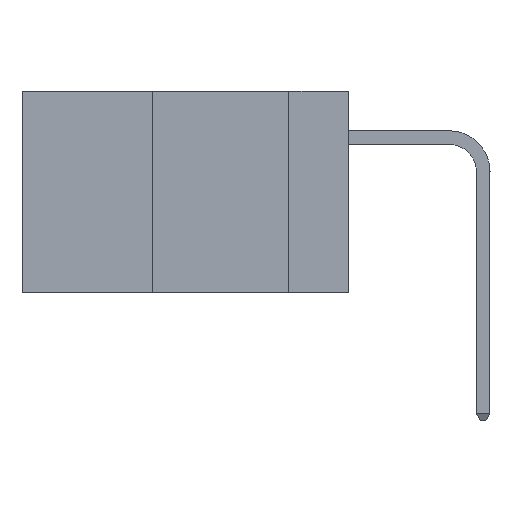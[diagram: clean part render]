
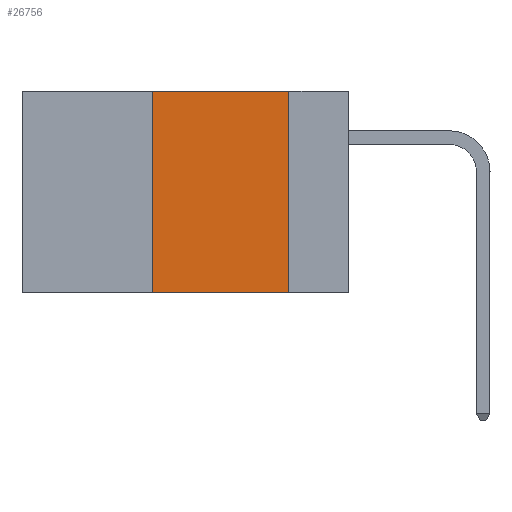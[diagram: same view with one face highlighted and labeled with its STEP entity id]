
A CAD part, left-side view. The second image highlights one B-rep face of the part: STEP entity #26756.
In plain terms, the highlighted planar face has unit normal (-1, 0, 0).
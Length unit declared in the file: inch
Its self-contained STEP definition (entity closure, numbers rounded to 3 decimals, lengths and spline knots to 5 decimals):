
#107 = CARTESIAN_POINT ( 'NONE',  ( 0., 0.11, 0. ) ) ;
#817 = VECTOR ( 'NONE', #8602, 39.37008 ) ;
#1219 = LINE ( 'NONE', #19257, #31223 ) ;
#3360 = VERTEX_POINT ( 'NONE', #4359 ) ;
#4359 = CARTESIAN_POINT ( 'NONE',  ( 0., 0.11, -0.37 ) ) ;
#5262 = CARTESIAN_POINT ( 'NONE',  ( 0., 0.6, -0.37 ) ) ;
#5291 = CARTESIAN_POINT ( 'NONE',  ( 0., 0.6, 0. ) ) ;
#7704 = EDGE_CURVE ( 'NONE', #17013, #25837, #30000, .T. ) ;
#8229 = DIRECTION ( 'NONE',  ( 0., 0., -1. ) ) ;
#8472 = ORIENTED_EDGE ( 'NONE', *, *, #32264, .T. ) ;
#8602 = DIRECTION ( 'NONE',  ( 0., -1., 0. ) ) ;
#11655 = VECTOR ( 'NONE', #19543, 39.37008 ) ;
#12601 = ORIENTED_EDGE ( 'NONE', *, *, #7704, .F. ) ;
#12730 = VERTEX_POINT ( 'NONE', #15192 ) ;
#12817 = CARTESIAN_POINT ( 'NONE',  ( 0., 0.11, 0. ) ) ;
#12995 = VECTOR ( 'NONE', #20111, 39.37008 ) ;
#13951 = EDGE_LOOP ( 'NONE', ( #27179, #12601, #33499, #8472 ) ) ;
#15192 = CARTESIAN_POINT ( 'NONE',  ( 0., 0.36, -0.37 ) ) ;
#17013 = VERTEX_POINT ( 'NONE', #19705 ) ;
#18565 = FACE_OUTER_BOUND ( 'NONE', #13951, .T. ) ;
#19257 = CARTESIAN_POINT ( 'NONE',  ( 0., 0.36, 0. ) ) ;
#19543 = DIRECTION ( 'NONE',  ( 0., -1., 0. ) ) ;
#19579 = PLANE ( 'NONE',  #21840 ) ;
#19705 = CARTESIAN_POINT ( 'NONE',  ( 0., 0.36, 0. ) ) ;
#20111 = DIRECTION ( 'NONE',  ( 0., 0., -1. ) ) ;
#20501 = LINE ( 'NONE', #107, #12995 ) ;
#21840 = AXIS2_PLACEMENT_3D ( 'NONE', #5291, #25158, #8229 ) ;
#25158 = DIRECTION ( 'NONE',  ( 1., 0., 0. ) ) ;
#25525 = CARTESIAN_POINT ( 'NONE',  ( 0., 0.6, 0. ) ) ;
#25837 = VERTEX_POINT ( 'NONE', #12817 ) ;
#26756 = ADVANCED_FACE ( 'NONE', ( #18565 ), #19579, .F. ) ;
#27179 = ORIENTED_EDGE ( 'NONE', *, *, #30407, .F. ) ;
#30000 = LINE ( 'NONE', #25525, #817 ) ;
#30407 = EDGE_CURVE ( 'NONE', #25837, #3360, #20501, .T. ) ;
#31223 = VECTOR ( 'NONE', #32987, 39.37008 ) ;
#32264 = EDGE_CURVE ( 'NONE', #12730, #3360, #33847, .T. ) ;
#32987 = DIRECTION ( 'NONE',  ( 0., 0., 1. ) ) ;
#33499 = ORIENTED_EDGE ( 'NONE', *, *, #34023, .F. ) ;
#33847 = LINE ( 'NONE', #5262, #11655 ) ;
#34023 = EDGE_CURVE ( 'NONE', #12730, #17013, #1219, .T. ) ;
